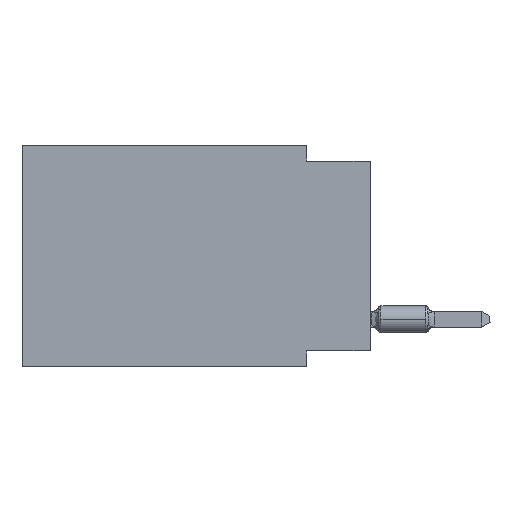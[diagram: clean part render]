
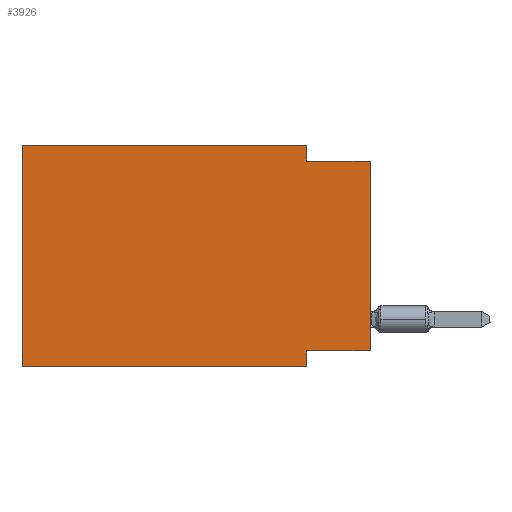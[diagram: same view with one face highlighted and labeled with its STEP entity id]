
A CAD part, left-side view. The second image highlights one B-rep face of the part: STEP entity #3926.
In plain terms, the highlighted planar face has unit normal (-1, 0, 0).
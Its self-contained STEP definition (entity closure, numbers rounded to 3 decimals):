
#3708 = DIRECTION ( 'NONE',  ( 0., -1., 0. ) ) ;
#3926 = ADVANCED_FACE ( 'NONE', ( #24110 ), #20035, .F. ) ;
#4392 = VERTEX_POINT ( 'NONE', #9889 ) ;
#4984 = CARTESIAN_POINT ( 'NONE',  ( 0., 13.97, 0. ) ) ;
#5673 = EDGE_CURVE ( 'NONE', #37509, #26219, #5791, .T. ) ;
#5791 = LINE ( 'NONE', #9883, #26837 ) ;
#6328 = VECTOR ( 'NONE', #6905, 1000. ) ;
#6614 = CARTESIAN_POINT ( 'NONE',  ( 0., 13.97, 0. ) ) ;
#6905 = DIRECTION ( 'NONE',  ( 0., 1., 0. ) ) ;
#7315 = CARTESIAN_POINT ( 'NONE',  ( 0., 13.97, 0. ) ) ;
#7943 = ORIENTED_EDGE ( 'NONE', *, *, #9846, .F. ) ;
#8130 = LINE ( 'NONE', #9505, #23922 ) ;
#8168 = VERTEX_POINT ( 'NONE', #40724 ) ;
#8547 = CARTESIAN_POINT ( 'NONE',  ( 0., 0., -0.635 ) ) ;
#8974 = VECTOR ( 'NONE', #10293, 1000. ) ;
#9505 = CARTESIAN_POINT ( 'NONE',  ( 0., 13.97, -8.89 ) ) ;
#9770 = ORIENTED_EDGE ( 'NONE', *, *, #22921, .F. ) ;
#9846 = EDGE_CURVE ( 'NONE', #44058, #10090, #32612, .T. ) ;
#9883 = CARTESIAN_POINT ( 'NONE',  ( 0., 0., -0.635 ) ) ;
#9889 = CARTESIAN_POINT ( 'NONE',  ( 0., 2.54, 0. ) ) ;
#10090 = VERTEX_POINT ( 'NONE', #45029 ) ;
#10293 = DIRECTION ( 'NONE',  ( 0., 0., -1. ) ) ;
#10527 = LINE ( 'NONE', #46991, #8974 ) ;
#13579 = DIRECTION ( 'NONE',  ( 0., -1., 0. ) ) ;
#14002 = ORIENTED_EDGE ( 'NONE', *, *, #23473, .F. ) ;
#14183 = VECTOR ( 'NONE', #29971, 1000. ) ;
#15561 = LINE ( 'NONE', #4984, #14183 ) ;
#16199 = VERTEX_POINT ( 'NONE', #46582 ) ;
#16962 = EDGE_LOOP ( 'NONE', ( #44024, #33363, #19712, #46656, #14002, #27432, #9770, #7943 ) ) ;
#17806 = DIRECTION ( 'NONE',  ( 0., 0., -1. ) ) ;
#17899 = AXIS2_PLACEMENT_3D ( 'NONE', #35399, #23873, #38524 ) ;
#18038 = LINE ( 'NONE', #29078, #21007 ) ;
#19712 = ORIENTED_EDGE ( 'NONE', *, *, #44853, .F. ) ;
#20035 = PLANE ( 'NONE',  #17899 ) ;
#20118 = EDGE_CURVE ( 'NONE', #8168, #16199, #8130, .T. ) ;
#20365 = EDGE_CURVE ( 'NONE', #36405, #4392, #39265, .T. ) ;
#20448 = DIRECTION ( 'NONE',  ( 0., -1., 0. ) ) ;
#21007 = VECTOR ( 'NONE', #17806, 1000. ) ;
#22921 = EDGE_CURVE ( 'NONE', #10090, #16199, #18038, .T. ) ;
#23473 = EDGE_CURVE ( 'NONE', #8168, #36405, #15561, .T. ) ;
#23873 = DIRECTION ( 'NONE',  ( 1., 0., 0. ) ) ;
#23922 = VECTOR ( 'NONE', #13579, 1000. ) ;
#24110 = FACE_OUTER_BOUND ( 'NONE', #16962, .T. ) ;
#24947 = LINE ( 'NONE', #43885, #39421 ) ;
#25106 = CARTESIAN_POINT ( 'NONE',  ( 0., 2.54, -0.635 ) ) ;
#26219 = VERTEX_POINT ( 'NONE', #8547 ) ;
#26837 = VECTOR ( 'NONE', #20448, 1000. ) ;
#27432 = ORIENTED_EDGE ( 'NONE', *, *, #20118, .T. ) ;
#27754 = EDGE_CURVE ( 'NONE', #44058, #26219, #24947, .T. ) ;
#28948 = CARTESIAN_POINT ( 'NONE',  ( 0., 0., -8.255 ) ) ;
#29078 = CARTESIAN_POINT ( 'NONE',  ( 0., 2.54, -8.89 ) ) ;
#29971 = DIRECTION ( 'NONE',  ( 0., 0., 1. ) ) ;
#32612 = LINE ( 'NONE', #33311, #6328 ) ;
#33311 = CARTESIAN_POINT ( 'NONE',  ( 0., 0., -8.255 ) ) ;
#33363 = ORIENTED_EDGE ( 'NONE', *, *, #5673, .F. ) ;
#35399 = CARTESIAN_POINT ( 'NONE',  ( 0., 13.97, 0. ) ) ;
#36224 = VECTOR ( 'NONE', #3708, 1000. ) ;
#36405 = VERTEX_POINT ( 'NONE', #6614 ) ;
#37509 = VERTEX_POINT ( 'NONE', #25106 ) ;
#38524 = DIRECTION ( 'NONE',  ( 0., 0., -1. ) ) ;
#39265 = LINE ( 'NONE', #7315, #36224 ) ;
#39421 = VECTOR ( 'NONE', #39594, 1000. ) ;
#39594 = DIRECTION ( 'NONE',  ( 0., 0., 1. ) ) ;
#40724 = CARTESIAN_POINT ( 'NONE',  ( 0., 13.97, -8.89 ) ) ;
#43885 = CARTESIAN_POINT ( 'NONE',  ( 0., 0., 0. ) ) ;
#44024 = ORIENTED_EDGE ( 'NONE', *, *, #27754, .T. ) ;
#44058 = VERTEX_POINT ( 'NONE', #28948 ) ;
#44853 = EDGE_CURVE ( 'NONE', #4392, #37509, #10527, .T. ) ;
#45029 = CARTESIAN_POINT ( 'NONE',  ( 0., 2.54, -8.255 ) ) ;
#46582 = CARTESIAN_POINT ( 'NONE',  ( 0., 2.54, -8.89 ) ) ;
#46656 = ORIENTED_EDGE ( 'NONE', *, *, #20365, .F. ) ;
#46991 = CARTESIAN_POINT ( 'NONE',  ( 0., 2.54, 0. ) ) ;
